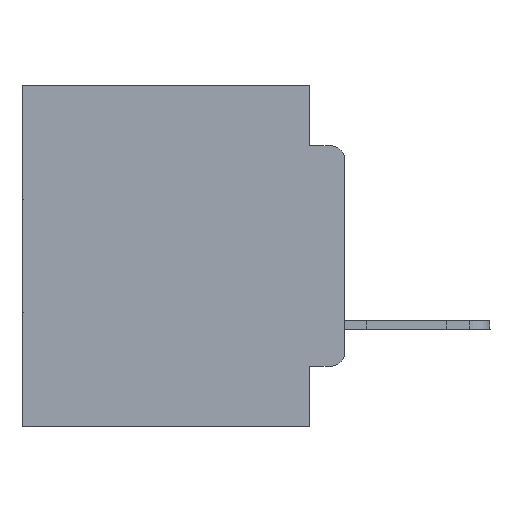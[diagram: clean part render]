
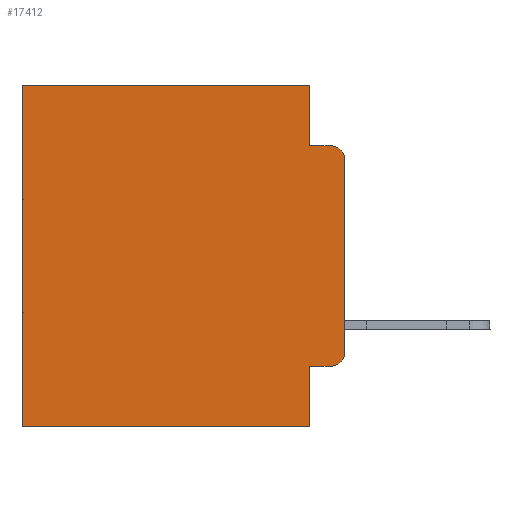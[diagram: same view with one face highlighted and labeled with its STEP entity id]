
A CAD part, left-side view. The second image highlights one B-rep face of the part: STEP entity #17412.
In plain terms, the highlighted planar face has unit normal (-1, 0, 0).
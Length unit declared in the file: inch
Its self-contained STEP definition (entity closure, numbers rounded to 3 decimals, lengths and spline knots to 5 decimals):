
#64 = CARTESIAN_POINT ( 'NONE',  ( 0.298, 0.051, -0.0885 ) ) ;
#107 = CARTESIAN_POINT ( 'NONE',  ( 0.298, 0.02, -0.4115 ) ) ;
#956 = CARTESIAN_POINT ( 'NONE',  ( 0.298, 0.051, -0.4115 ) ) ;
#1113 = ORIENTED_EDGE ( 'NONE', *, *, #13066, .F. ) ;
#2166 = CARTESIAN_POINT ( 'NONE',  ( 0.298, 0., -0.1085 ) ) ;
#2931 = CARTESIAN_POINT ( 'NONE',  ( 0.298, 0., -0.3915 ) ) ;
#3013 = EDGE_CURVE ( 'NONE', #19147, #14520, #12036, .T. ) ;
#3291 = DIRECTION ( 'NONE',  ( 0., 1., 0. ) ) ;
#3293 = DIRECTION ( 'NONE',  ( 0., 0., -1. ) ) ;
#3991 = AXIS2_PLACEMENT_3D ( 'NONE', #29432, #12365, #8720 ) ;
#5567 = FACE_OUTER_BOUND ( 'NONE', #7139, .T. ) ;
#5786 = DIRECTION ( 'NONE',  ( -1., 0., 0. ) ) ;
#6214 = EDGE_CURVE ( 'NONE', #24657, #28452, #27560, .T. ) ;
#6383 = CIRCLE ( 'NONE', #3991, 0.02 ) ;
#6892 = EDGE_CURVE ( 'NONE', #24115, #24657, #10259, .T. ) ;
#7011 = VECTOR ( 'NONE', #20035, 39.37008 ) ;
#7139 = EDGE_LOOP ( 'NONE', ( #16655, #29273, #1113, #11548, #14877, #15016, #7954, #18672, #19731, #18574 ) ) ;
#7579 = CARTESIAN_POINT ( 'NONE',  ( 0.298, 0.051, -0.5 ) ) ;
#7648 = LINE ( 'NONE', #22120, #28115 ) ;
#7854 = CARTESIAN_POINT ( 'NONE',  ( 0.298, 0., 0. ) ) ;
#7954 = ORIENTED_EDGE ( 'NONE', *, *, #28681, .F. ) ;
#8551 = LINE ( 'NONE', #24709, #7011 ) ;
#8578 = CARTESIAN_POINT ( 'NONE',  ( 0.298, 0.051, -0.4115 ) ) ;
#8713 = AXIS2_PLACEMENT_3D ( 'NONE', #21990, #5786, #24551 ) ;
#8720 = DIRECTION ( 'NONE',  ( 0., 0., -1. ) ) ;
#9230 = LINE ( 'NONE', #20882, #26186 ) ;
#9457 = CARTESIAN_POINT ( 'NONE',  ( 0.298, 0.051, 0. ) ) ;
#9634 = VERTEX_POINT ( 'NONE', #11622 ) ;
#9902 = LINE ( 'NONE', #956, #26735 ) ;
#10002 = EDGE_CURVE ( 'NONE', #23281, #28656, #6383, .T. ) ;
#10111 = PLANE ( 'NONE',  #20860 ) ;
#10259 = LINE ( 'NONE', #12360, #21771 ) ;
#10614 = DIRECTION ( 'NONE',  ( 0., 1., 0. ) ) ;
#10935 = CARTESIAN_POINT ( 'NONE',  ( 0.298, 0.473, 0. ) ) ;
#11547 = VECTOR ( 'NONE', #13323, 39.37008 ) ;
#11548 = ORIENTED_EDGE ( 'NONE', *, *, #28894, .F. ) ;
#11622 = CARTESIAN_POINT ( 'NONE',  ( 0.298, 0.051, -0.0885 ) ) ;
#11997 = EDGE_CURVE ( 'NONE', #18539, #12416, #27762, .T. ) ;
#12036 = CIRCLE ( 'NONE', #8713, 0.02 ) ;
#12360 = CARTESIAN_POINT ( 'NONE',  ( 0.298, 0., 0. ) ) ;
#12365 = DIRECTION ( 'NONE',  ( -1., 0., 0. ) ) ;
#12416 = VERTEX_POINT ( 'NONE', #7579 ) ;
#13066 = EDGE_CURVE ( 'NONE', #9634, #14520, #27169, .T. ) ;
#13323 = DIRECTION ( 'NONE',  ( 0., 0., -1. ) ) ;
#14520 = VERTEX_POINT ( 'NONE', #19222 ) ;
#14877 = ORIENTED_EDGE ( 'NONE', *, *, #6892, .T. ) ;
#15016 = ORIENTED_EDGE ( 'NONE', *, *, #6214, .T. ) ;
#15098 = VECTOR ( 'NONE', #18682, 39.37008 ) ;
#16655 = ORIENTED_EDGE ( 'NONE', *, *, #22348, .F. ) ;
#16669 = VECTOR ( 'NONE', #24903, 39.37008 ) ;
#16706 = DIRECTION ( 'NONE',  ( 0., -1., 0. ) ) ;
#17412 = ADVANCED_FACE ( 'NONE', ( #5567 ), #10111, .F. ) ;
#18539 = VERTEX_POINT ( 'NONE', #8578 ) ;
#18574 = ORIENTED_EDGE ( 'NONE', *, *, #10002, .T. ) ;
#18672 = ORIENTED_EDGE ( 'NONE', *, *, #11997, .F. ) ;
#18682 = DIRECTION ( 'NONE',  ( 0., 0., -1. ) ) ;
#18865 = EDGE_CURVE ( 'NONE', #18539, #23281, #9902, .T. ) ;
#19056 = DIRECTION ( 'NONE',  ( 0., 0., -1. ) ) ;
#19147 = VERTEX_POINT ( 'NONE', #2166 ) ;
#19222 = CARTESIAN_POINT ( 'NONE',  ( 0.298, 0.02, -0.0885 ) ) ;
#19731 = ORIENTED_EDGE ( 'NONE', *, *, #18865, .T. ) ;
#20035 = DIRECTION ( 'NONE',  ( 0., 0., -1. ) ) ;
#20860 = AXIS2_PLACEMENT_3D ( 'NONE', #7854, #21316, #3293 ) ;
#20882 = CARTESIAN_POINT ( 'NONE',  ( 0.298, 0.051, 0. ) ) ;
#21316 = DIRECTION ( 'NONE',  ( 1., 0., 0. ) ) ;
#21771 = VECTOR ( 'NONE', #3291, 39.37008 ) ;
#21990 = CARTESIAN_POINT ( 'NONE',  ( 0.298, 0.02, -0.1085 ) ) ;
#22120 = CARTESIAN_POINT ( 'NONE',  ( 0.298, 0., -0.5 ) ) ;
#22348 = EDGE_CURVE ( 'NONE', #19147, #28656, #8551, .T. ) ;
#22937 = CARTESIAN_POINT ( 'NONE',  ( 0.298, 0.473, -0.5 ) ) ;
#23131 = CARTESIAN_POINT ( 'NONE',  ( 0.298, 0.473, 0. ) ) ;
#23281 = VERTEX_POINT ( 'NONE', #107 ) ;
#24115 = VERTEX_POINT ( 'NONE', #27407 ) ;
#24551 = DIRECTION ( 'NONE',  ( 0., 0., -1. ) ) ;
#24657 = VERTEX_POINT ( 'NONE', #23131 ) ;
#24709 = CARTESIAN_POINT ( 'NONE',  ( 0.298, 0., 0. ) ) ;
#24903 = DIRECTION ( 'NONE',  ( 0., -1., 0. ) ) ;
#26186 = VECTOR ( 'NONE', #19056, 39.37008 ) ;
#26735 = VECTOR ( 'NONE', #16706, 39.37008 ) ;
#27169 = LINE ( 'NONE', #64, #16669 ) ;
#27407 = CARTESIAN_POINT ( 'NONE',  ( 0.298, 0.051, 0. ) ) ;
#27560 = LINE ( 'NONE', #10935, #11547 ) ;
#27762 = LINE ( 'NONE', #9457, #15098 ) ;
#28115 = VECTOR ( 'NONE', #10614, 39.37008 ) ;
#28452 = VERTEX_POINT ( 'NONE', #22937 ) ;
#28656 = VERTEX_POINT ( 'NONE', #2931 ) ;
#28681 = EDGE_CURVE ( 'NONE', #12416, #28452, #7648, .T. ) ;
#28894 = EDGE_CURVE ( 'NONE', #24115, #9634, #9230, .T. ) ;
#29273 = ORIENTED_EDGE ( 'NONE', *, *, #3013, .T. ) ;
#29432 = CARTESIAN_POINT ( 'NONE',  ( 0.298, 0.02, -0.3915 ) ) ;
